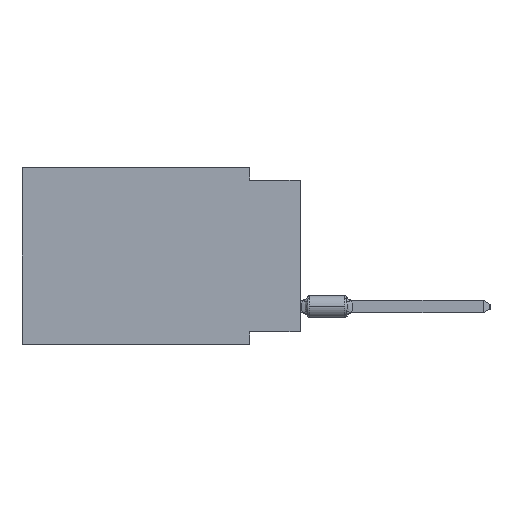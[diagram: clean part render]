
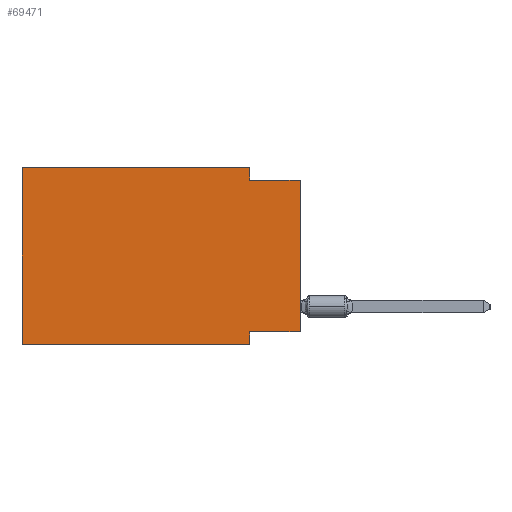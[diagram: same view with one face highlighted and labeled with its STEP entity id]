
A CAD part, left-side view. The second image highlights one B-rep face of the part: STEP entity #69471.
In plain terms, the highlighted planar face has unit normal (-1, 0, 0).
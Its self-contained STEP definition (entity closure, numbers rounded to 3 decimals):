
#1147 = DIRECTION ( 'NONE',  ( 0., 0., -1. ) ) ;
#1691 = CARTESIAN_POINT ( 'NONE',  ( 0., 13.97, 0. ) ) ;
#2428 = EDGE_LOOP ( 'NONE', ( #6154, #32229, #91353, #20635, #59135, #16710, #53813, #64977 ) ) ;
#2564 = VERTEX_POINT ( 'NONE', #34716 ) ;
#3856 = CARTESIAN_POINT ( 'NONE',  ( 0., 0., -8.255 ) ) ;
#4679 = VERTEX_POINT ( 'NONE', #52066 ) ;
#5831 = EDGE_CURVE ( 'NONE', #21377, #92803, #7829, .T. ) ;
#6154 = ORIENTED_EDGE ( 'NONE', *, *, #82711, .T. ) ;
#6684 = LINE ( 'NONE', #31412, #81615 ) ;
#7829 = LINE ( 'NONE', #39952, #95897 ) ;
#7926 = CARTESIAN_POINT ( 'NONE',  ( 0., 13.97, 0. ) ) ;
#9004 = VERTEX_POINT ( 'NONE', #77784 ) ;
#16710 = ORIENTED_EDGE ( 'NONE', *, *, #92427, .T. ) ;
#17498 = DIRECTION ( 'NONE',  ( 0., 0., -1. ) ) ;
#18853 = LINE ( 'NONE', #83625, #30477 ) ;
#20208 = DIRECTION ( 'NONE',  ( 0., 0., 1. ) ) ;
#20210 = VECTOR ( 'NONE', #1147, 1000. ) ;
#20635 = ORIENTED_EDGE ( 'NONE', *, *, #73600, .F. ) ;
#21377 = VERTEX_POINT ( 'NONE', #44458 ) ;
#28961 = EDGE_CURVE ( 'NONE', #53544, #21377, #62302, .T. ) ;
#30291 = CARTESIAN_POINT ( 'NONE',  ( 0., 0., -0.635 ) ) ;
#30477 = VECTOR ( 'NONE', #74683, 1000. ) ;
#31412 = CARTESIAN_POINT ( 'NONE',  ( 0., 13.97, 0. ) ) ;
#31444 = VERTEX_POINT ( 'NONE', #30291 ) ;
#32229 = ORIENTED_EDGE ( 'NONE', *, *, #69859, .F. ) ;
#34716 = CARTESIAN_POINT ( 'NONE',  ( 0., 13.97, 0. ) ) ;
#37033 = EDGE_CURVE ( 'NONE', #88156, #9004, #66962, .T. ) ;
#37466 = VECTOR ( 'NONE', #64283, 1000. ) ;
#38064 = DIRECTION ( 'NONE',  ( 0., 1., 0. ) ) ;
#39952 = CARTESIAN_POINT ( 'NONE',  ( 0., 2.54, -8.89 ) ) ;
#41569 = EDGE_CURVE ( 'NONE', #4679, #2564, #6684, .T. ) ;
#44458 = CARTESIAN_POINT ( 'NONE',  ( 0., 2.54, -8.255 ) ) ;
#50678 = AXIS2_PLACEMENT_3D ( 'NONE', #1691, #67501, #17498 ) ;
#51063 = LINE ( 'NONE', #82656, #102744 ) ;
#52066 = CARTESIAN_POINT ( 'NONE',  ( 0., 13.97, -8.89 ) ) ;
#53544 = VERTEX_POINT ( 'NONE', #54595 ) ;
#53813 = ORIENTED_EDGE ( 'NONE', *, *, #5831, .F. ) ;
#54595 = CARTESIAN_POINT ( 'NONE',  ( 0., 0., -8.255 ) ) ;
#56293 = DIRECTION ( 'NONE',  ( 0., 0., -1. ) ) ;
#58443 = VECTOR ( 'NONE', #38064, 1000. ) ;
#58579 = FACE_OUTER_BOUND ( 'NONE', #2428, .T. ) ;
#59135 = ORIENTED_EDGE ( 'NONE', *, *, #41569, .F. ) ;
#59539 = VECTOR ( 'NONE', #20208, 1000. ) ;
#62302 = LINE ( 'NONE', #3856, #58443 ) ;
#63549 = DIRECTION ( 'NONE',  ( 0., 0., 1. ) ) ;
#64283 = DIRECTION ( 'NONE',  ( 0., -1., 0. ) ) ;
#64977 = ORIENTED_EDGE ( 'NONE', *, *, #28961, .F. ) ;
#65638 = CARTESIAN_POINT ( 'NONE',  ( 0., 2.54, -8.89 ) ) ;
#66099 = LINE ( 'NONE', #98214, #59539 ) ;
#66962 = LINE ( 'NONE', #97000, #20210 ) ;
#67501 = DIRECTION ( 'NONE',  ( 1., 0., 0. ) ) ;
#69471 = ADVANCED_FACE ( 'NONE', ( #58579 ), #82780, .F. ) ;
#69859 = EDGE_CURVE ( 'NONE', #9004, #31444, #51063, .T. ) ;
#73600 = EDGE_CURVE ( 'NONE', #2564, #88156, #80080, .T. ) ;
#74683 = DIRECTION ( 'NONE',  ( 0., -1., 0. ) ) ;
#77784 = CARTESIAN_POINT ( 'NONE',  ( 0., 2.54, -0.635 ) ) ;
#80080 = LINE ( 'NONE', #7926, #37466 ) ;
#81615 = VECTOR ( 'NONE', #63549, 1000. ) ;
#82656 = CARTESIAN_POINT ( 'NONE',  ( 0., 0., -0.635 ) ) ;
#82711 = EDGE_CURVE ( 'NONE', #53544, #31444, #66099, .T. ) ;
#82780 = PLANE ( 'NONE',  #50678 ) ;
#83625 = CARTESIAN_POINT ( 'NONE',  ( 0., 13.97, -8.89 ) ) ;
#88156 = VERTEX_POINT ( 'NONE', #96074 ) ;
#91075 = DIRECTION ( 'NONE',  ( 0., -1., 0. ) ) ;
#91353 = ORIENTED_EDGE ( 'NONE', *, *, #37033, .F. ) ;
#92427 = EDGE_CURVE ( 'NONE', #4679, #92803, #18853, .T. ) ;
#92803 = VERTEX_POINT ( 'NONE', #65638 ) ;
#95897 = VECTOR ( 'NONE', #56293, 1000. ) ;
#96074 = CARTESIAN_POINT ( 'NONE',  ( 0., 2.54, 0. ) ) ;
#97000 = CARTESIAN_POINT ( 'NONE',  ( 0., 2.54, 0. ) ) ;
#98214 = CARTESIAN_POINT ( 'NONE',  ( 0., 0., 0. ) ) ;
#102744 = VECTOR ( 'NONE', #91075, 1000. ) ;
